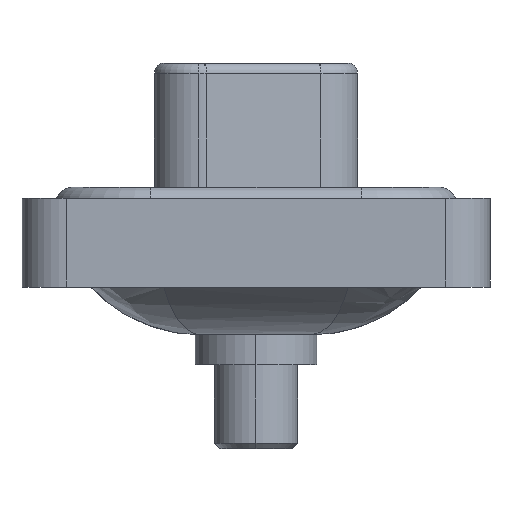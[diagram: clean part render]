
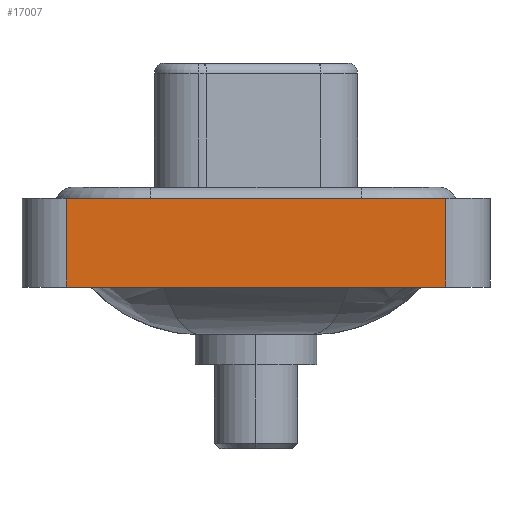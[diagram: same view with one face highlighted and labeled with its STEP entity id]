
A CAD part, left-side view. The second image highlights one B-rep face of the part: STEP entity #17007.
In plain terms, the highlighted planar face has unit normal (-1, 0, 0).
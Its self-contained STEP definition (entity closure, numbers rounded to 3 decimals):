
#142 = ORIENTED_EDGE ( 'NONE', *, *, #9726, .F. ) ;
#354 = DIRECTION ( 'NONE',  ( 0., 0., 1. ) ) ;
#582 = CARTESIAN_POINT ( 'NONE',  ( -7.35, -8.55, 0.4 ) ) ;
#736 = DIRECTION ( 'NONE',  ( 0., 0., 1. ) ) ;
#762 = VERTEX_POINT ( 'NONE', #16169 ) ;
#1121 = FACE_OUTER_BOUND ( 'NONE', #11037, .T. ) ;
#2135 = CARTESIAN_POINT ( 'NONE',  ( -7.35, 8.55, -3.6 ) ) ;
#2957 = EDGE_CURVE ( 'NONE', #5958, #7697, #17205, .T. ) ;
#3630 = CARTESIAN_POINT ( 'NONE',  ( -7.35, 8.55, -3.6 ) ) ;
#3747 = PLANE ( 'NONE',  #16096 ) ;
#4941 = VECTOR ( 'NONE', #354, 1000. ) ;
#5351 = EDGE_CURVE ( 'NONE', #762, #15545, #12657, .T. ) ;
#5958 = VERTEX_POINT ( 'NONE', #2135 ) ;
#6360 = LINE ( 'NONE', #16127, #9940 ) ;
#6458 = CARTESIAN_POINT ( 'NONE',  ( -7.35, -8.55, -3.6 ) ) ;
#6550 = DIRECTION ( 'NONE',  ( 0., -1., 0. ) ) ;
#7697 = VERTEX_POINT ( 'NONE', #8385 ) ;
#8385 = CARTESIAN_POINT ( 'NONE',  ( -7.35, 8.55, 0.4 ) ) ;
#8633 = LINE ( 'NONE', #582, #15750 ) ;
#9726 = EDGE_CURVE ( 'NONE', #7697, #15545, #8633, .T. ) ;
#9940 = VECTOR ( 'NONE', #6550, 1000. ) ;
#10376 = CARTESIAN_POINT ( 'NONE',  ( -7.35, -8.55, 0.4 ) ) ;
#10435 = ORIENTED_EDGE ( 'NONE', *, *, #2957, .F. ) ;
#10989 = ORIENTED_EDGE ( 'NONE', *, *, #13755, .T. ) ;
#11037 = EDGE_LOOP ( 'NONE', ( #15951, #142, #10435, #10989 ) ) ;
#11977 = DIRECTION ( 'NONE',  ( -1., 0., 0. ) ) ;
#12657 = LINE ( 'NONE', #13916, #4941 ) ;
#13421 = DIRECTION ( 'NONE',  ( 0., 0., 1. ) ) ;
#13755 = EDGE_CURVE ( 'NONE', #5958, #762, #6360, .T. ) ;
#13916 = CARTESIAN_POINT ( 'NONE',  ( -7.35, -8.55, -3.6 ) ) ;
#14142 = DIRECTION ( 'NONE',  ( 0., -1., 0. ) ) ;
#14429 = VECTOR ( 'NONE', #736, 1000. ) ;
#15545 = VERTEX_POINT ( 'NONE', #10376 ) ;
#15750 = VECTOR ( 'NONE', #14142, 1000. ) ;
#15951 = ORIENTED_EDGE ( 'NONE', *, *, #5351, .T. ) ;
#16096 = AXIS2_PLACEMENT_3D ( 'NONE', #6458, #11977, #13421 ) ;
#16127 = CARTESIAN_POINT ( 'NONE',  ( -7.35, -8.55, -3.6 ) ) ;
#16169 = CARTESIAN_POINT ( 'NONE',  ( -7.35, -8.55, -3.6 ) ) ;
#17007 = ADVANCED_FACE ( 'NONE', ( #1121 ), #3747, .T. ) ;
#17205 = LINE ( 'NONE', #3630, #14429 ) ;
